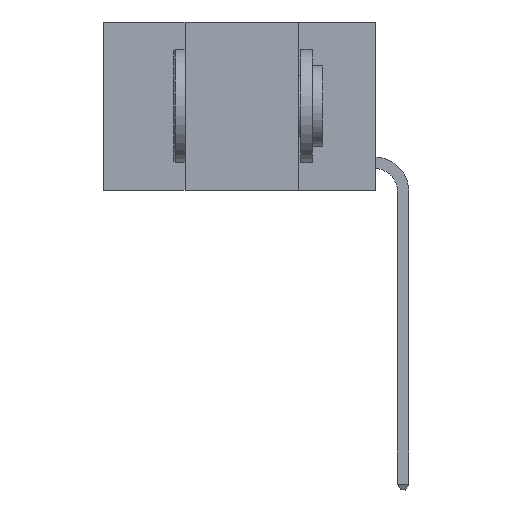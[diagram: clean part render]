
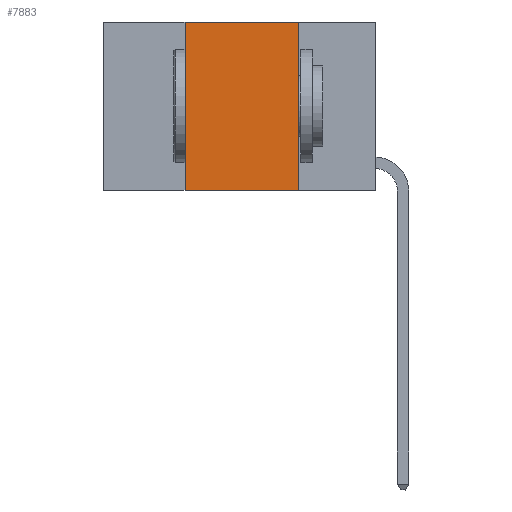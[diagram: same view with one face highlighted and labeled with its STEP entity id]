
A CAD part, left-side view. The second image highlights one B-rep face of the part: STEP entity #7883.
In plain terms, the highlighted planar face has unit normal (-1, 0, 0).
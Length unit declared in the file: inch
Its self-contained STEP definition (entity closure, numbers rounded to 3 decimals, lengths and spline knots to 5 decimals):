
#304 = DIRECTION ( 'NONE',  ( 0., -1., 0. ) ) ;
#1533 = DIRECTION ( 'NONE',  ( 0., -1., 0. ) ) ;
#1549 = CARTESIAN_POINT ( 'NONE',  ( 0., 0.6, 0. ) ) ;
#1589 = DIRECTION ( 'NONE',  ( 1., 0., 0. ) ) ;
#1609 = ORIENTED_EDGE ( 'NONE', *, *, #10438, .T. ) ;
#1618 = VECTOR ( 'NONE', #304, 39.37008 ) ;
#2715 = FACE_OUTER_BOUND ( 'NONE', #13812, .T. ) ;
#3084 = LINE ( 'NONE', #6954, #7505 ) ;
#3759 = EDGE_CURVE ( 'NONE', #7254, #13841, #16258, .T. ) ;
#4192 = VERTEX_POINT ( 'NONE', #16628 ) ;
#4214 = VECTOR ( 'NONE', #1533, 39.37008 ) ;
#5532 = LINE ( 'NONE', #18441, #9392 ) ;
#6051 = AXIS2_PLACEMENT_3D ( 'NONE', #21012, #1589, #13186 ) ;
#6136 = EDGE_CURVE ( 'NONE', #13841, #4192, #3084, .T. ) ;
#6954 = CARTESIAN_POINT ( 'NONE',  ( 0., 0.17, 0. ) ) ;
#7254 = VERTEX_POINT ( 'NONE', #14517 ) ;
#7505 = VECTOR ( 'NONE', #18270, 39.37008 ) ;
#7883 = ADVANCED_FACE ( 'NONE', ( #2715 ), #9880, .F. ) ;
#8629 = CARTESIAN_POINT ( 'NONE',  ( 0., 0.6, -0.37 ) ) ;
#9392 = VECTOR ( 'NONE', #12127, 39.37008 ) ;
#9880 = PLANE ( 'NONE',  #6051 ) ;
#10438 = EDGE_CURVE ( 'NONE', #19283, #4192, #19435, .T. ) ;
#10503 = EDGE_CURVE ( 'NONE', #19283, #7254, #5532, .T. ) ;
#11844 = CARTESIAN_POINT ( 'NONE',  ( 0., 0.17, 0. ) ) ;
#12127 = DIRECTION ( 'NONE',  ( 0., 0., 1. ) ) ;
#13186 = DIRECTION ( 'NONE',  ( 0., 0., -1. ) ) ;
#13812 = EDGE_LOOP ( 'NONE', ( #14174, #14616, #14667, #1609 ) ) ;
#13841 = VERTEX_POINT ( 'NONE', #11844 ) ;
#14174 = ORIENTED_EDGE ( 'NONE', *, *, #6136, .F. ) ;
#14517 = CARTESIAN_POINT ( 'NONE',  ( 0., 0.42, 0. ) ) ;
#14616 = ORIENTED_EDGE ( 'NONE', *, *, #3759, .F. ) ;
#14667 = ORIENTED_EDGE ( 'NONE', *, *, #10503, .F. ) ;
#15926 = CARTESIAN_POINT ( 'NONE',  ( 0., 0.42, -0.37 ) ) ;
#16258 = LINE ( 'NONE', #1549, #4214 ) ;
#16628 = CARTESIAN_POINT ( 'NONE',  ( 0., 0.17, -0.37 ) ) ;
#18270 = DIRECTION ( 'NONE',  ( 0., 0., -1. ) ) ;
#18441 = CARTESIAN_POINT ( 'NONE',  ( 0., 0.42, 0. ) ) ;
#19283 = VERTEX_POINT ( 'NONE', #15926 ) ;
#19435 = LINE ( 'NONE', #8629, #1618 ) ;
#21012 = CARTESIAN_POINT ( 'NONE',  ( 0., 0.6, 0. ) ) ;
